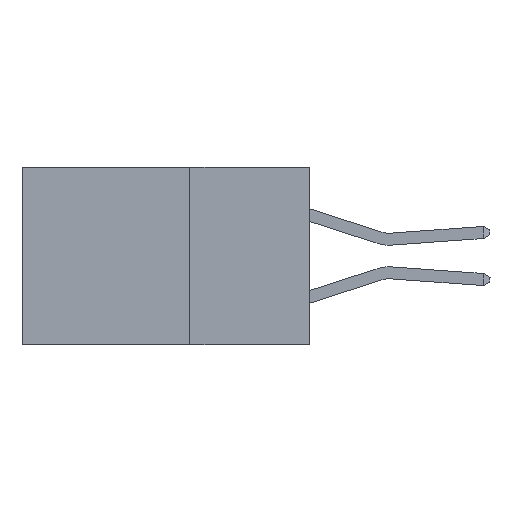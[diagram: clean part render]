
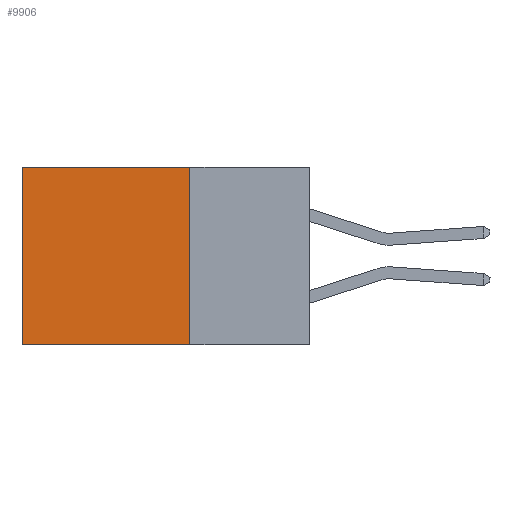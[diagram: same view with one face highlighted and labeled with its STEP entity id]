
A CAD part, left-side view. The second image highlights one B-rep face of the part: STEP entity #9906.
In plain terms, the highlighted planar face has unit normal (-1, 0, 0).
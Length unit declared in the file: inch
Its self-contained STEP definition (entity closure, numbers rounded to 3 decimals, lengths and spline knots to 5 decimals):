
#195 = EDGE_CURVE ( 'NONE', #5743, #1005, #12858, .T. ) ;
#1005 = VERTEX_POINT ( 'NONE', #10873 ) ;
#1076 = EDGE_LOOP ( 'NONE', ( #11126, #6213, #14590, #4235 ) ) ;
#3022 = AXIS2_PLACEMENT_3D ( 'NONE', #7585, #5210, #13722 ) ;
#3203 = CARTESIAN_POINT ( 'NONE',  ( 0.298, 0.6, 0. ) ) ;
#3232 = CARTESIAN_POINT ( 'NONE',  ( 0.298, 0.25, -0.37 ) ) ;
#4235 = ORIENTED_EDGE ( 'NONE', *, *, #12109, .T. ) ;
#5210 = DIRECTION ( 'NONE',  ( 1., 0., 0. ) ) ;
#5743 = VERTEX_POINT ( 'NONE', #12827 ) ;
#5794 = VECTOR ( 'NONE', #15005, 39.37008 ) ;
#5831 = VECTOR ( 'NONE', #13080, 39.37008 ) ;
#5950 = EDGE_CURVE ( 'NONE', #11985, #14019, #12861, .T. ) ;
#6213 = ORIENTED_EDGE ( 'NONE', *, *, #11299, .F. ) ;
#7585 = CARTESIAN_POINT ( 'NONE',  ( 0.298, 0.25, 0. ) ) ;
#9056 = LINE ( 'NONE', #3232, #5831 ) ;
#9732 = CARTESIAN_POINT ( 'NONE',  ( 0.298, 0.25, 0. ) ) ;
#9906 = ADVANCED_FACE ( 'NONE', ( #12196 ), #13658, .F. ) ;
#10873 = CARTESIAN_POINT ( 'NONE',  ( 0.298, 0.6, -0.37 ) ) ;
#11000 = VECTOR ( 'NONE', #14582, 39.37008 ) ;
#11126 = ORIENTED_EDGE ( 'NONE', *, *, #195, .T. ) ;
#11299 = EDGE_CURVE ( 'NONE', #14019, #1005, #9056, .T. ) ;
#11477 = CARTESIAN_POINT ( 'NONE',  ( 0.298, 0.25, 0. ) ) ;
#11985 = VERTEX_POINT ( 'NONE', #14643 ) ;
#12109 = EDGE_CURVE ( 'NONE', #11985, #5743, #12657, .T. ) ;
#12196 = FACE_OUTER_BOUND ( 'NONE', #1076, .T. ) ;
#12657 = LINE ( 'NONE', #11477, #5794 ) ;
#12790 = DIRECTION ( 'NONE',  ( 0., 0., -1. ) ) ;
#12827 = CARTESIAN_POINT ( 'NONE',  ( 0.298, 0.6, 0. ) ) ;
#12858 = LINE ( 'NONE', #3203, #14763 ) ;
#12861 = LINE ( 'NONE', #9732, #11000 ) ;
#13080 = DIRECTION ( 'NONE',  ( 0., 1., 0. ) ) ;
#13658 = PLANE ( 'NONE',  #3022 ) ;
#13722 = DIRECTION ( 'NONE',  ( 0., 0., -1. ) ) ;
#14019 = VERTEX_POINT ( 'NONE', #15550 ) ;
#14582 = DIRECTION ( 'NONE',  ( 0., 0., -1. ) ) ;
#14590 = ORIENTED_EDGE ( 'NONE', *, *, #5950, .F. ) ;
#14643 = CARTESIAN_POINT ( 'NONE',  ( 0.298, 0.25, 0. ) ) ;
#14763 = VECTOR ( 'NONE', #12790, 39.37008 ) ;
#15005 = DIRECTION ( 'NONE',  ( 0., 1., 0. ) ) ;
#15550 = CARTESIAN_POINT ( 'NONE',  ( 0.298, 0.25, -0.37 ) ) ;
